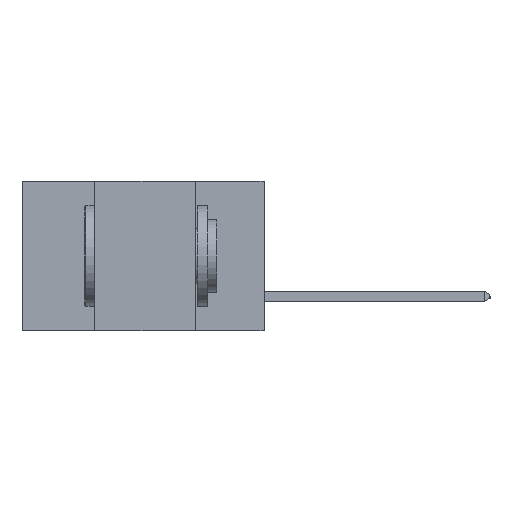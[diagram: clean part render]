
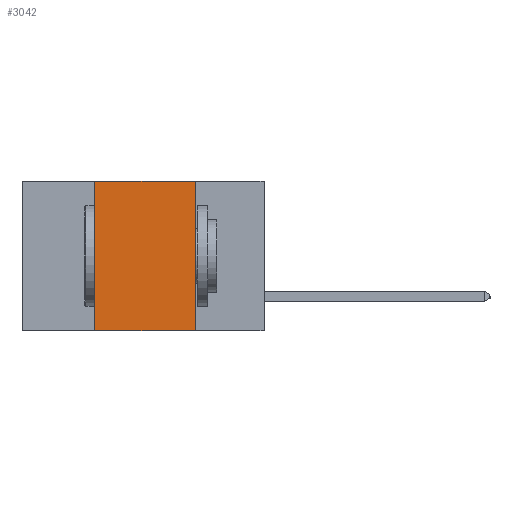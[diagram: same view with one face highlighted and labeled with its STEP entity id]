
A CAD part, left-side view. The second image highlights one B-rep face of the part: STEP entity #3042.
In plain terms, the highlighted planar face has unit normal (-1, 0, 0).
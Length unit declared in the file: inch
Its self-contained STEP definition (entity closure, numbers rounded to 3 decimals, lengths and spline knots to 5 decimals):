
#4 = PLANE ( 'NONE',  #2413 ) ;
#1981 = VERTEX_POINT ( 'NONE', #9894 ) ;
#2413 = AXIS2_PLACEMENT_3D ( 'NONE', #9345, #2584, #9312 ) ;
#2584 = DIRECTION ( 'NONE',  ( 1., 0., 0. ) ) ;
#2983 = EDGE_CURVE ( 'NONE', #1981, #7327, #6383, .T. ) ;
#3039 = EDGE_CURVE ( 'NONE', #7327, #8937, #11517, .T. ) ;
#3042 = ADVANCED_FACE ( 'NONE', ( #8287 ), #4, .F. ) ;
#5336 = VECTOR ( 'NONE', #9714, 39.37008 ) ;
#5585 = LINE ( 'NONE', #8769, #13852 ) ;
#5934 = ORIENTED_EDGE ( 'NONE', *, *, #12605, .F. ) ;
#6043 = VECTOR ( 'NONE', #11458, 39.37008 ) ;
#6383 = LINE ( 'NONE', #11421, #6043 ) ;
#7123 = LINE ( 'NONE', #8935, #12528 ) ;
#7327 = VERTEX_POINT ( 'NONE', #12822 ) ;
#7489 = ORIENTED_EDGE ( 'NONE', *, *, #3039, .F. ) ;
#8287 = FACE_OUTER_BOUND ( 'NONE', #10192, .T. ) ;
#8688 = CARTESIAN_POINT ( 'NONE',  ( 0., 0.17, -0.37 ) ) ;
#8769 = CARTESIAN_POINT ( 'NONE',  ( 0., 0.6, -0.37 ) ) ;
#8935 = CARTESIAN_POINT ( 'NONE',  ( 0., 0.17, 0. ) ) ;
#8937 = VERTEX_POINT ( 'NONE', #12331 ) ;
#9312 = DIRECTION ( 'NONE',  ( 0., 0., -1. ) ) ;
#9345 = CARTESIAN_POINT ( 'NONE',  ( 0., 0.6, 0. ) ) ;
#9604 = VERTEX_POINT ( 'NONE', #8688 ) ;
#9700 = CARTESIAN_POINT ( 'NONE',  ( 0., 0.6, 0. ) ) ;
#9710 = ORIENTED_EDGE ( 'NONE', *, *, #12094, .T. ) ;
#9714 = DIRECTION ( 'NONE',  ( 0., -1., 0. ) ) ;
#9894 = CARTESIAN_POINT ( 'NONE',  ( 0., 0.42, -0.37 ) ) ;
#10069 = DIRECTION ( 'NONE',  ( 0., 0., -1. ) ) ;
#10192 = EDGE_LOOP ( 'NONE', ( #5934, #7489, #10611, #9710 ) ) ;
#10611 = ORIENTED_EDGE ( 'NONE', *, *, #2983, .F. ) ;
#11421 = CARTESIAN_POINT ( 'NONE',  ( 0., 0.42, 0. ) ) ;
#11458 = DIRECTION ( 'NONE',  ( 0., 0., 1. ) ) ;
#11517 = LINE ( 'NONE', #9700, #5336 ) ;
#12094 = EDGE_CURVE ( 'NONE', #1981, #9604, #5585, .T. ) ;
#12331 = CARTESIAN_POINT ( 'NONE',  ( 0., 0.17, 0. ) ) ;
#12528 = VECTOR ( 'NONE', #10069, 39.37008 ) ;
#12605 = EDGE_CURVE ( 'NONE', #8937, #9604, #7123, .T. ) ;
#12822 = CARTESIAN_POINT ( 'NONE',  ( 0., 0.42, 0. ) ) ;
#12975 = DIRECTION ( 'NONE',  ( 0., -1., 0. ) ) ;
#13852 = VECTOR ( 'NONE', #12975, 39.37008 ) ;
